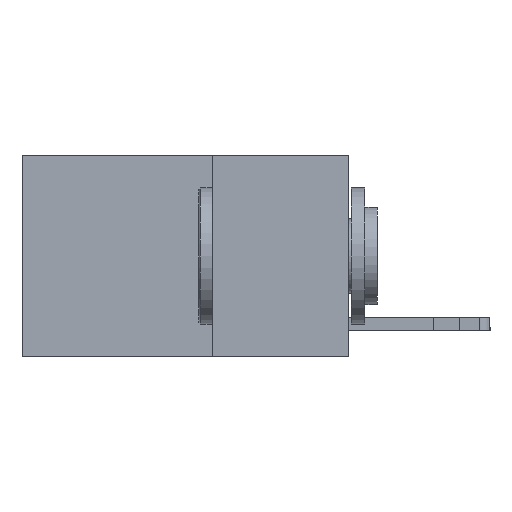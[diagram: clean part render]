
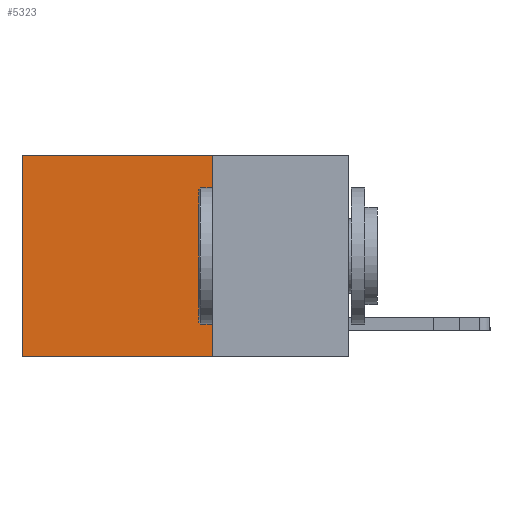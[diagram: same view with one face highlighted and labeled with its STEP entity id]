
A CAD part, left-side view. The second image highlights one B-rep face of the part: STEP entity #5323.
In plain terms, the highlighted planar face has unit normal (-1, 0, 0).
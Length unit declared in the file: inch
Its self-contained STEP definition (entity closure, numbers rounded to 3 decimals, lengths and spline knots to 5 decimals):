
#239 = VECTOR ( 'NONE', #12639, 39.37008 ) ;
#465 = EDGE_CURVE ( 'NONE', #2163, #9753, #13185, .T. ) ;
#876 = CARTESIAN_POINT ( 'NONE',  ( 0.2625, 0.25, -0.37 ) ) ;
#1814 = VECTOR ( 'NONE', #15523, 39.37008 ) ;
#1951 = VERTEX_POINT ( 'NONE', #16566 ) ;
#2163 = VERTEX_POINT ( 'NONE', #3556 ) ;
#3219 = CARTESIAN_POINT ( 'NONE',  ( 0.2625, 0.6, -0.37 ) ) ;
#3556 = CARTESIAN_POINT ( 'NONE',  ( 0.2625, 0.25, 0. ) ) ;
#3953 = LINE ( 'NONE', #9777, #1814 ) ;
#4032 = DIRECTION ( 'NONE',  ( 0., 0., -1. ) ) ;
#4389 = FACE_OUTER_BOUND ( 'NONE', #12142, .T. ) ;
#5104 = VECTOR ( 'NONE', #7568, 39.37008 ) ;
#5236 = EDGE_CURVE ( 'NONE', #9753, #16818, #5360, .T. ) ;
#5323 = ADVANCED_FACE ( 'NONE', ( #4389 ), #5814, .F. ) ;
#5360 = LINE ( 'NONE', #876, #239 ) ;
#5814 = PLANE ( 'NONE',  #11216 ) ;
#6267 = VECTOR ( 'NONE', #17676, 39.37008 ) ;
#7565 = EDGE_CURVE ( 'NONE', #1951, #16818, #3953, .T. ) ;
#7568 = DIRECTION ( 'NONE',  ( 0., 1., 0. ) ) ;
#7605 = ORIENTED_EDGE ( 'NONE', *, *, #13828, .T. ) ;
#9316 = ORIENTED_EDGE ( 'NONE', *, *, #465, .F. ) ;
#9753 = VERTEX_POINT ( 'NONE', #13950 ) ;
#9777 = CARTESIAN_POINT ( 'NONE',  ( 0.2625, 0.6, 0. ) ) ;
#10352 = ORIENTED_EDGE ( 'NONE', *, *, #7565, .T. ) ;
#11216 = AXIS2_PLACEMENT_3D ( 'NONE', #13182, #14625, #4032 ) ;
#11851 = CARTESIAN_POINT ( 'NONE',  ( 0.2625, 0.25, 0. ) ) ;
#12142 = EDGE_LOOP ( 'NONE', ( #10352, #14438, #9316, #7605 ) ) ;
#12639 = DIRECTION ( 'NONE',  ( 0., 1., 0. ) ) ;
#13182 = CARTESIAN_POINT ( 'NONE',  ( 0.2625, 0.25, 0. ) ) ;
#13185 = LINE ( 'NONE', #11851, #6267 ) ;
#13828 = EDGE_CURVE ( 'NONE', #2163, #1951, #14657, .T. ) ;
#13950 = CARTESIAN_POINT ( 'NONE',  ( 0.2625, 0.25, -0.37 ) ) ;
#14204 = CARTESIAN_POINT ( 'NONE',  ( 0.2625, 0.25, 0. ) ) ;
#14438 = ORIENTED_EDGE ( 'NONE', *, *, #5236, .F. ) ;
#14625 = DIRECTION ( 'NONE',  ( 1., 0., 0. ) ) ;
#14657 = LINE ( 'NONE', #14204, #5104 ) ;
#15523 = DIRECTION ( 'NONE',  ( 0., 0., -1. ) ) ;
#16566 = CARTESIAN_POINT ( 'NONE',  ( 0.2625, 0.6, 0. ) ) ;
#16818 = VERTEX_POINT ( 'NONE', #3219 ) ;
#17676 = DIRECTION ( 'NONE',  ( 0., 0., -1. ) ) ;
